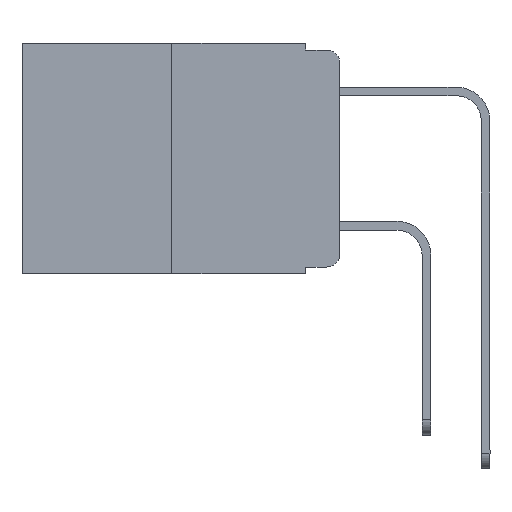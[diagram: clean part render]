
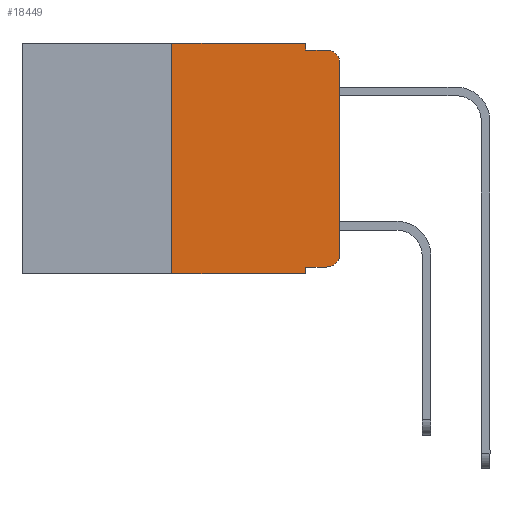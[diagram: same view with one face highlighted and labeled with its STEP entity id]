
A CAD part, left-side view. The second image highlights one B-rep face of the part: STEP entity #18449.
In plain terms, the highlighted planar face has unit normal (-1, 0, 0).
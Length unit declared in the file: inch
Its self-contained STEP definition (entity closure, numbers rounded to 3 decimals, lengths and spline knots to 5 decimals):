
#83 = VERTEX_POINT ( 'NONE', #8768 ) ;
#180 = PLANE ( 'NONE',  #2201 ) ;
#239 = VECTOR ( 'NONE', #17714, 39.37008 ) ;
#709 = ORIENTED_EDGE ( 'NONE', *, *, #9340, .T. ) ;
#1121 = CIRCLE ( 'NONE', #4154, 0.02 ) ;
#1411 = VERTEX_POINT ( 'NONE', #20804 ) ;
#1571 = ORIENTED_EDGE ( 'NONE', *, *, #7145, .T. ) ;
#2131 = CARTESIAN_POINT ( 'NONE',  ( 0., 0., 0. ) ) ;
#2201 = AXIS2_PLACEMENT_3D ( 'NONE', #9876, #7995, #20757 ) ;
#2556 = DIRECTION ( 'NONE',  ( 0., -1., 0. ) ) ;
#2749 = DIRECTION ( 'NONE',  ( 0., 0., -1. ) ) ;
#3190 = DIRECTION ( 'NONE',  ( -1., 0., 0. ) ) ;
#3191 = LINE ( 'NONE', #9616, #17247 ) ;
#3731 = ORIENTED_EDGE ( 'NONE', *, *, #10297, .T. ) ;
#3916 = LINE ( 'NONE', #12237, #20297 ) ;
#3956 = LINE ( 'NONE', #10271, #12648 ) ;
#4084 = VERTEX_POINT ( 'NONE', #16901 ) ;
#4154 = AXIS2_PLACEMENT_3D ( 'NONE', #16399, #19573, #8394 ) ;
#4575 = EDGE_CURVE ( 'NONE', #1411, #19087, #12343, .T. ) ;
#4955 = CARTESIAN_POINT ( 'NONE',  ( 0., 0.02, -0.01 ) ) ;
#5075 = CARTESIAN_POINT ( 'NONE',  ( 0., 0.051, -0.01 ) ) ;
#5200 = LINE ( 'NONE', #15417, #19575 ) ;
#5294 = CARTESIAN_POINT ( 'NONE',  ( 0., 0.051, 0. ) ) ;
#5362 = ORIENTED_EDGE ( 'NONE', *, *, #8237, .F. ) ;
#5862 = AXIS2_PLACEMENT_3D ( 'NONE', #11423, #3190, #8242 ) ;
#6183 = VERTEX_POINT ( 'NONE', #5075 ) ;
#6576 = ORIENTED_EDGE ( 'NONE', *, *, #4575, .T. ) ;
#7145 = EDGE_CURVE ( 'NONE', #4084, #83, #5200, .T. ) ;
#7205 = CARTESIAN_POINT ( 'NONE',  ( 0., 0., -0.03 ) ) ;
#7898 = CIRCLE ( 'NONE', #5862, 0.02 ) ;
#7995 = DIRECTION ( 'NONE',  ( 1., 0., 0. ) ) ;
#8237 = EDGE_CURVE ( 'NONE', #17212, #20829, #15335, .T. ) ;
#8242 = DIRECTION ( 'NONE',  ( 0., 0., -1. ) ) ;
#8394 = DIRECTION ( 'NONE',  ( 0., 0., -1. ) ) ;
#8671 = EDGE_CURVE ( 'NONE', #6183, #9017, #3916, .T. ) ;
#8768 = CARTESIAN_POINT ( 'NONE',  ( 0., 0.02, -0.333 ) ) ;
#9017 = VERTEX_POINT ( 'NONE', #4955 ) ;
#9063 = DIRECTION ( 'NONE',  ( 0., -1., 0. ) ) ;
#9340 = EDGE_CURVE ( 'NONE', #83, #1411, #1121, .T. ) ;
#9379 = VERTEX_POINT ( 'NONE', #9765 ) ;
#9605 = CARTESIAN_POINT ( 'NONE',  ( 0., 0.051, 0. ) ) ;
#9616 = CARTESIAN_POINT ( 'NONE',  ( 0., 0.473, -0.343 ) ) ;
#9765 = CARTESIAN_POINT ( 'NONE',  ( 0., 0.25, -0.343 ) ) ;
#9819 = DIRECTION ( 'NONE',  ( 0., -1., 0. ) ) ;
#9876 = CARTESIAN_POINT ( 'NONE',  ( 0., 0.473, 0. ) ) ;
#10167 = DIRECTION ( 'NONE',  ( 0., 0., 1. ) ) ;
#10271 = CARTESIAN_POINT ( 'NONE',  ( 0., 0.25, 0. ) ) ;
#10297 = EDGE_CURVE ( 'NONE', #19087, #9017, #7898, .T. ) ;
#10541 = ORIENTED_EDGE ( 'NONE', *, *, #16302, .T. ) ;
#10738 = EDGE_LOOP ( 'NONE', ( #6576, #3731, #15006, #19639, #5362, #13923, #10541, #12719, #1571, #709 ) ) ;
#11423 = CARTESIAN_POINT ( 'NONE',  ( 0., 0.02, -0.03 ) ) ;
#11697 = CARTESIAN_POINT ( 'NONE',  ( 0., 0.25, 0. ) ) ;
#11778 = CARTESIAN_POINT ( 'NONE',  ( 0., 0.473, 0. ) ) ;
#12237 = CARTESIAN_POINT ( 'NONE',  ( 0., 0.051, -0.01 ) ) ;
#12343 = LINE ( 'NONE', #2131, #20553 ) ;
#12648 = VECTOR ( 'NONE', #10167, 39.37008 ) ;
#12719 = ORIENTED_EDGE ( 'NONE', *, *, #14485, .F. ) ;
#12815 = CARTESIAN_POINT ( 'NONE',  ( 0., 0.051, -0.343 ) ) ;
#13446 = DIRECTION ( 'NONE',  ( 0., -1., 0. ) ) ;
#13923 = ORIENTED_EDGE ( 'NONE', *, *, #19063, .F. ) ;
#14020 = DIRECTION ( 'NONE',  ( 0., 0., 1. ) ) ;
#14485 = EDGE_CURVE ( 'NONE', #4084, #17515, #14569, .T. ) ;
#14569 = LINE ( 'NONE', #9605, #239 ) ;
#14891 = VECTOR ( 'NONE', #13446, 39.37008 ) ;
#15006 = ORIENTED_EDGE ( 'NONE', *, *, #8671, .F. ) ;
#15335 = LINE ( 'NONE', #11778, #14891 ) ;
#15417 = CARTESIAN_POINT ( 'NONE',  ( 0., 0.051, -0.333 ) ) ;
#16302 = EDGE_CURVE ( 'NONE', #9379, #17515, #3191, .T. ) ;
#16399 = CARTESIAN_POINT ( 'NONE',  ( 0., 0.02, -0.313 ) ) ;
#16695 = VECTOR ( 'NONE', #2749, 39.37008 ) ;
#16901 = CARTESIAN_POINT ( 'NONE',  ( 0., 0.051, -0.333 ) ) ;
#17183 = CARTESIAN_POINT ( 'NONE',  ( 0., 0.051, 0. ) ) ;
#17212 = VERTEX_POINT ( 'NONE', #11697 ) ;
#17247 = VECTOR ( 'NONE', #9819, 39.37008 ) ;
#17515 = VERTEX_POINT ( 'NONE', #12815 ) ;
#17714 = DIRECTION ( 'NONE',  ( 0., 0., -1. ) ) ;
#17785 = FACE_OUTER_BOUND ( 'NONE', #10738, .T. ) ;
#18449 = ADVANCED_FACE ( 'NONE', ( #17785 ), #180, .F. ) ;
#18664 = LINE ( 'NONE', #17183, #16695 ) ;
#19063 = EDGE_CURVE ( 'NONE', #9379, #17212, #3956, .T. ) ;
#19087 = VERTEX_POINT ( 'NONE', #7205 ) ;
#19573 = DIRECTION ( 'NONE',  ( -1., 0., 0. ) ) ;
#19575 = VECTOR ( 'NONE', #2556, 39.37008 ) ;
#19598 = EDGE_CURVE ( 'NONE', #20829, #6183, #18664, .T. ) ;
#19639 = ORIENTED_EDGE ( 'NONE', *, *, #19598, .F. ) ;
#20297 = VECTOR ( 'NONE', #9063, 39.37008 ) ;
#20553 = VECTOR ( 'NONE', #14020, 39.37008 ) ;
#20757 = DIRECTION ( 'NONE',  ( 0., 0., -1. ) ) ;
#20804 = CARTESIAN_POINT ( 'NONE',  ( 0., 0., -0.313 ) ) ;
#20829 = VERTEX_POINT ( 'NONE', #5294 ) ;
